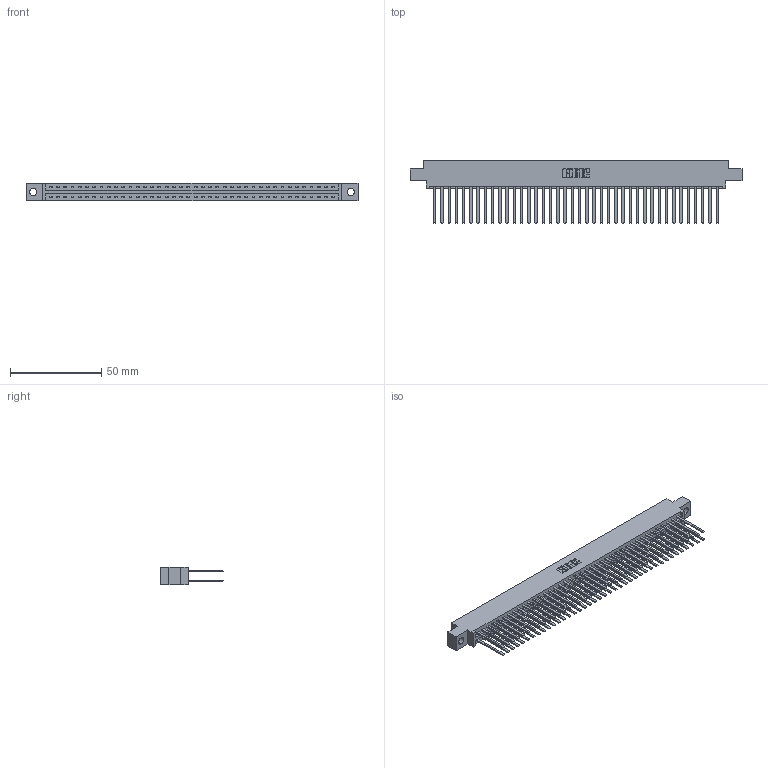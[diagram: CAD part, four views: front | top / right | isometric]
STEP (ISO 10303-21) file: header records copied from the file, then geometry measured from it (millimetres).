
FILE_DESCRIPTION (( 'STEP AP203' ), '1' );
FILE_NAME ('387-080-544-804.STEP', '2018-09-23T18:52:50', ( '' ), ( '' ), 'SwSTEP 2.0', 'SolidWorks 2016', '' );
FILE_SCHEMA (( 'CONFIG_CONTROL_DESIGN' ));
Length unit declared in the file: inch
Products named in the file (3): 345-292-001_345-293-144; 387-080-544-804; 337 Part_0.170 Offset - 0.156 Dia-TH
Assembly tree (81 placements, depth 2):
  387-080-544-804
    337 Part_0.170 Offset - 0.156 Dia-TH
    345-292-001_345-293-144  x80
Bounding box: 181.51 x 34.3 x 9.4 mm (x, y, z)
Volume: 20018.3 mm3; surface area: 26180 mm2
Topology: 81 solids, 81 shells, 3958 faces, 11763 edges, 7734 vertices
Faces by surface type: plane 2794, cylinder 1164
Entity records: 31223 total; most frequent: CARTESIAN_POINT 5262, ORIENTED_EDGE 5198, DIRECTION 4475, EDGE_CURVE 2599, VECTOR 2475, LINE 2475, VERTEX_POINT 1730, AXIS2_PLACEMENT_3D 1000
